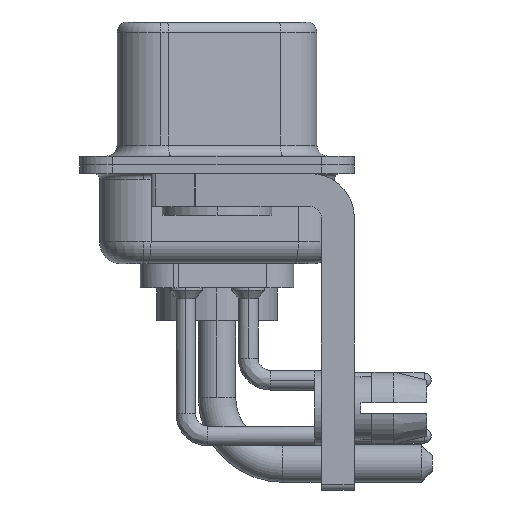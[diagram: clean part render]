
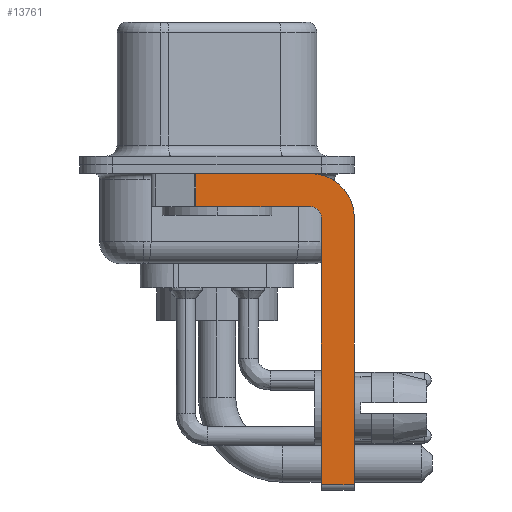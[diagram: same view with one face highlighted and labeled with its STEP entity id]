
A CAD part, left-side view. The second image highlights one B-rep face of the part: STEP entity #13761.
In plain terms, the highlighted planar face has unit normal (-1, 0, 0).
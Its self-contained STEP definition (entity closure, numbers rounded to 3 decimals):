
#184 = EDGE_CURVE ( 'NONE', #3162, #7836, #6202, .T. ) ;
#204 = LINE ( 'NONE', #14984, #19062 ) ;
#420 = CARTESIAN_POINT ( 'NONE',  ( -2.9, -4.25, -0.4 ) ) ;
#1268 = DIRECTION ( 'NONE',  ( 0., 0., -1. ) ) ;
#1531 = CIRCLE ( 'NONE', #8726, 2. ) ;
#1678 = CARTESIAN_POINT ( 'NONE',  ( -2.9, -4.75, -2.4 ) ) ;
#2781 = CARTESIAN_POINT ( 'NONE',  ( -2.9, -4.75, -14.8 ) ) ;
#3146 = DIRECTION ( 'NONE',  ( 1., 0., 0. ) ) ;
#3162 = VERTEX_POINT ( 'NONE', #12722 ) ;
#3197 = CARTESIAN_POINT ( 'NONE',  ( -2.9, -6.25, -14.55 ) ) ;
#4116 = VECTOR ( 'NONE', #5012, 1000. ) ;
#4615 = PLANE ( 'NONE',  #13786 ) ;
#4698 = DIRECTION ( 'NONE',  ( 0., 0., 1. ) ) ;
#5012 = DIRECTION ( 'NONE',  ( 0., -1., 0. ) ) ;
#5502 = VECTOR ( 'NONE', #18552, 1000. ) ;
#6159 = LINE ( 'NONE', #19427, #13192 ) ;
#6202 = LINE ( 'NONE', #8082, #24344 ) ;
#6580 = CARTESIAN_POINT ( 'NONE',  ( -2.9, -4.25, -2.4 ) ) ;
#6904 = LINE ( 'NONE', #2781, #23481 ) ;
#7147 = ORIENTED_EDGE ( 'NONE', *, *, #12041, .T. ) ;
#7425 = CARTESIAN_POINT ( 'NONE',  ( -2.9, -4.25, -1.9 ) ) ;
#7604 = VERTEX_POINT ( 'NONE', #1678 ) ;
#7836 = VERTEX_POINT ( 'NONE', #420 ) ;
#7993 = EDGE_CURVE ( 'NONE', #16704, #7604, #6904, .T. ) ;
#8082 = CARTESIAN_POINT ( 'NONE',  ( -2.9, 3., -0.4 ) ) ;
#8083 = CARTESIAN_POINT ( 'NONE',  ( -2.9, -4.25, -2.4 ) ) ;
#8726 = AXIS2_PLACEMENT_3D ( 'NONE', #8083, #3146, #1268 ) ;
#9931 = VERTEX_POINT ( 'NONE', #3197 ) ;
#10121 = FACE_OUTER_BOUND ( 'NONE', #13775, .T. ) ;
#10629 = EDGE_CURVE ( 'NONE', #11891, #15259, #6159, .T. ) ;
#10653 = CIRCLE ( 'NONE', #16277, 0.5 ) ;
#11735 = ORIENTED_EDGE ( 'NONE', *, *, #10629, .F. ) ;
#11891 = VERTEX_POINT ( 'NONE', #7425 ) ;
#12041 = EDGE_CURVE ( 'NONE', #16704, #9931, #21814, .T. ) ;
#12246 = CARTESIAN_POINT ( 'NONE',  ( -2.9, -4.25, -2.4 ) ) ;
#12722 = CARTESIAN_POINT ( 'NONE',  ( -2.9, 0.978, -0.4 ) ) ;
#13192 = VECTOR ( 'NONE', #21565, 1000. ) ;
#13388 = VERTEX_POINT ( 'NONE', #16661 ) ;
#13761 = ADVANCED_FACE ( 'NONE', ( #10121 ), #4615, .F. ) ;
#13775 = EDGE_LOOP ( 'NONE', ( #15725, #21746, #11735, #13915, #19697, #7147, #16828, #20416 ) ) ;
#13786 = AXIS2_PLACEMENT_3D ( 'NONE', #12246, #19898, #15523 ) ;
#13915 = ORIENTED_EDGE ( 'NONE', *, *, #24085, .F. ) ;
#14215 = DIRECTION ( 'NONE',  ( -1., 0., 0. ) ) ;
#14984 = CARTESIAN_POINT ( 'NONE',  ( -2.9, -6.25, -2.4 ) ) ;
#15259 = VERTEX_POINT ( 'NONE', #21582 ) ;
#15523 = DIRECTION ( 'NONE',  ( 0., 0., -1. ) ) ;
#15725 = ORIENTED_EDGE ( 'NONE', *, *, #184, .F. ) ;
#16277 = AXIS2_PLACEMENT_3D ( 'NONE', #6580, #14215, #4698 ) ;
#16539 = DIRECTION ( 'NONE',  ( 0., 0., 1. ) ) ;
#16661 = CARTESIAN_POINT ( 'NONE',  ( -2.9, -6.25, -2.4 ) ) ;
#16678 = CARTESIAN_POINT ( 'NONE',  ( -2.9, 0.978, -1.9 ) ) ;
#16704 = VERTEX_POINT ( 'NONE', #22260 ) ;
#16828 = ORIENTED_EDGE ( 'NONE', *, *, #18172, .F. ) ;
#18172 = EDGE_CURVE ( 'NONE', #13388, #9931, #204, .T. ) ;
#18552 = DIRECTION ( 'NONE',  ( 0., 0., -1. ) ) ;
#18869 = DIRECTION ( 'NONE',  ( 0., 0., -1. ) ) ;
#19062 = VECTOR ( 'NONE', #18869, 1000. ) ;
#19427 = CARTESIAN_POINT ( 'NONE',  ( -2.9, -4.25, -1.9 ) ) ;
#19697 = ORIENTED_EDGE ( 'NONE', *, *, #7993, .F. ) ;
#19898 = DIRECTION ( 'NONE',  ( 1., 0., 0. ) ) ;
#20416 = ORIENTED_EDGE ( 'NONE', *, *, #21550, .F. ) ;
#20937 = LINE ( 'NONE', #16678, #5502 ) ;
#21550 = EDGE_CURVE ( 'NONE', #7836, #13388, #1531, .T. ) ;
#21565 = DIRECTION ( 'NONE',  ( 0., 1., 0. ) ) ;
#21582 = CARTESIAN_POINT ( 'NONE',  ( -2.9, 0.978, -1.9 ) ) ;
#21746 = ORIENTED_EDGE ( 'NONE', *, *, #24540, .T. ) ;
#21814 = LINE ( 'NONE', #22185, #4116 ) ;
#22185 = CARTESIAN_POINT ( 'NONE',  ( -2.9, -4.25, -14.55 ) ) ;
#22260 = CARTESIAN_POINT ( 'NONE',  ( -2.9, -4.75, -14.55 ) ) ;
#23123 = DIRECTION ( 'NONE',  ( 0., -1., 0. ) ) ;
#23481 = VECTOR ( 'NONE', #16539, 1000. ) ;
#24085 = EDGE_CURVE ( 'NONE', #7604, #11891, #10653, .T. ) ;
#24344 = VECTOR ( 'NONE', #23123, 1000. ) ;
#24540 = EDGE_CURVE ( 'NONE', #3162, #15259, #20937, .T. ) ;
